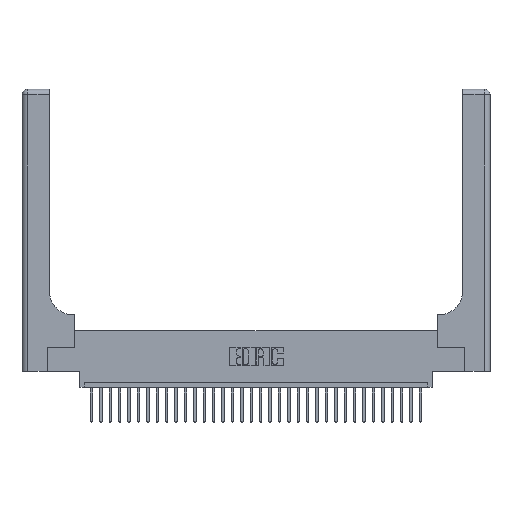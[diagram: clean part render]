
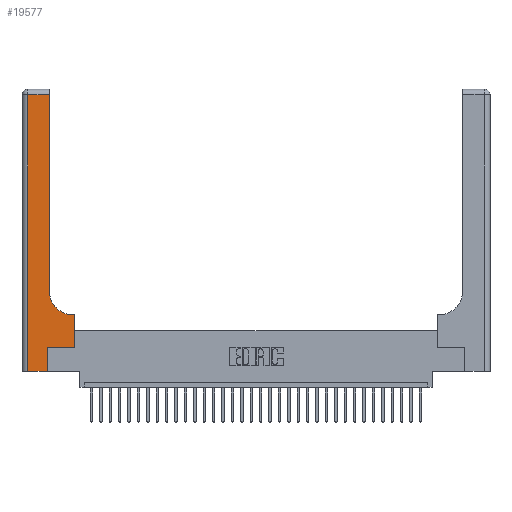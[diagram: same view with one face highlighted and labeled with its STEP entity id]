
A CAD part, top view. The second image highlights one B-rep face of the part: STEP entity #19577.
In plain terms, the highlighted planar face has unit normal (0, 0, 1).
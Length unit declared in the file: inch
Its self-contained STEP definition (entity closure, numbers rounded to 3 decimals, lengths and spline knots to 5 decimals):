
#452 = CARTESIAN_POINT ( 'NONE',  ( 0.5415, 0.6, 0.37 ) ) ;
#463 = VERTEX_POINT ( 'NONE', #10119 ) ;
#527 = CARTESIAN_POINT ( 'NONE',  ( 0.2915, 0.85, 0.37 ) ) ;
#620 = LINE ( 'NONE', #13643, #3871 ) ;
#786 = CARTESIAN_POINT ( 'NONE',  ( 0., 0., 0.37 ) ) ;
#1481 = LINE ( 'NONE', #9128, #20385 ) ;
#1831 = EDGE_CURVE ( 'NONE', #19878, #11481, #620, .T. ) ;
#1938 = CARTESIAN_POINT ( 'NONE',  ( 0.269, 0.25, 0.37 ) ) ;
#2171 = DIRECTION ( 'NONE',  ( 1., 0., 0. ) ) ;
#2666 = ORIENTED_EDGE ( 'NONE', *, *, #7732, .T. ) ;
#2807 = VECTOR ( 'NONE', #29113, 39.37008 ) ;
#3871 = VECTOR ( 'NONE', #11151, 39.37008 ) ;
#4984 = CIRCLE ( 'NONE', #26012, 0.25 ) ;
#5066 = LINE ( 'NONE', #786, #33152 ) ;
#5218 = DIRECTION ( 'NONE',  ( -1., 0., 0. ) ) ;
#6144 = VECTOR ( 'NONE', #14206, 39.37008 ) ;
#7732 = EDGE_CURVE ( 'NONE', #9405, #19878, #31428, .T. ) ;
#7807 = DIRECTION ( 'NONE',  ( 0., 0., -1. ) ) ;
#8270 = EDGE_CURVE ( 'NONE', #23010, #9405, #9745, .T. ) ;
#8709 = EDGE_CURVE ( 'NONE', #11481, #463, #5066, .T. ) ;
#9128 = CARTESIAN_POINT ( 'NONE',  ( 0.5585, 0.25, 0.37 ) ) ;
#9405 = VERTEX_POINT ( 'NONE', #33171 ) ;
#9745 = LINE ( 'NONE', #11195, #2807 ) ;
#10119 = CARTESIAN_POINT ( 'NONE',  ( 0.269, 0., 0.37 ) ) ;
#10226 = EDGE_CURVE ( 'NONE', #18715, #23010, #4984, .T. ) ;
#10331 = PLANE ( 'NONE',  #28315 ) ;
#10439 = ORIENTED_EDGE ( 'NONE', *, *, #27239, .T. ) ;
#11151 = DIRECTION ( 'NONE',  ( 0., -1., 0. ) ) ;
#11195 = CARTESIAN_POINT ( 'NONE',  ( 0.2915, 3., 0.37 ) ) ;
#11481 = VERTEX_POINT ( 'NONE', #20960 ) ;
#12913 = ORIENTED_EDGE ( 'NONE', *, *, #24461, .T. ) ;
#13223 = LINE ( 'NONE', #31880, #21623 ) ;
#13295 = ORIENTED_EDGE ( 'NONE', *, *, #23652, .T. ) ;
#13319 = CARTESIAN_POINT ( 'NONE',  ( 0.269, 0.25, 0.37 ) ) ;
#13643 = CARTESIAN_POINT ( 'NONE',  ( 0.06, 3., 0.37 ) ) ;
#14206 = DIRECTION ( 'NONE',  ( -1., 0., 0. ) ) ;
#14352 = EDGE_CURVE ( 'NONE', #16293, #25494, #1481, .T. ) ;
#15084 = CARTESIAN_POINT ( 'NONE',  ( 0.5585, 0.6, 0.37 ) ) ;
#15350 = ORIENTED_EDGE ( 'NONE', *, *, #10226, .T. ) ;
#15387 = EDGE_LOOP ( 'NONE', ( #16786, #2666, #30426, #17628, #10439, #12913, #19989, #13295, #15350 ) ) ;
#16293 = VERTEX_POINT ( 'NONE', #30199 ) ;
#16786 = ORIENTED_EDGE ( 'NONE', *, *, #8270, .T. ) ;
#16866 = CARTESIAN_POINT ( 'NONE',  ( 0., 2.94, 0.37 ) ) ;
#17628 = ORIENTED_EDGE ( 'NONE', *, *, #8709, .T. ) ;
#17678 = CARTESIAN_POINT ( 'NONE',  ( 0.06, 2.94, 0.37 ) ) ;
#18127 = FACE_OUTER_BOUND ( 'NONE', #15387, .T. ) ;
#18715 = VERTEX_POINT ( 'NONE', #452 ) ;
#19284 = CARTESIAN_POINT ( 'NONE',  ( 0.5415, 0.85, 0.37 ) ) ;
#19577 = ADVANCED_FACE ( 'NONE', ( #18127 ), #10331, .F. ) ;
#19878 = VERTEX_POINT ( 'NONE', #17678 ) ;
#19989 = ORIENTED_EDGE ( 'NONE', *, *, #14352, .T. ) ;
#20385 = VECTOR ( 'NONE', #22114, 39.37008 ) ;
#20569 = CARTESIAN_POINT ( 'NONE',  ( 0., 3., 0.37 ) ) ;
#20960 = CARTESIAN_POINT ( 'NONE',  ( 0.06, 0., 0.37 ) ) ;
#21623 = VECTOR ( 'NONE', #26392, 39.37008 ) ;
#21866 = DIRECTION ( 'NONE',  ( 0., 0., -1. ) ) ;
#22114 = DIRECTION ( 'NONE',  ( 0., 1., 0. ) ) ;
#22216 = LINE ( 'NONE', #13319, #23031 ) ;
#23010 = VERTEX_POINT ( 'NONE', #527 ) ;
#23031 = VECTOR ( 'NONE', #26514, 39.37008 ) ;
#23652 = EDGE_CURVE ( 'NONE', #25494, #18715, #28240, .T. ) ;
#24461 = EDGE_CURVE ( 'NONE', #31440, #16293, #22216, .T. ) ;
#25494 = VERTEX_POINT ( 'NONE', #15084 ) ;
#26012 = AXIS2_PLACEMENT_3D ( 'NONE', #19284, #21866, #2171 ) ;
#26392 = DIRECTION ( 'NONE',  ( 0., 1., 0. ) ) ;
#26514 = DIRECTION ( 'NONE',  ( 1., 0., 0. ) ) ;
#26657 = DIRECTION ( 'NONE',  ( -1., 0., 0. ) ) ;
#26867 = DIRECTION ( 'NONE',  ( 1., 0., 0. ) ) ;
#27239 = EDGE_CURVE ( 'NONE', #463, #31440, #13223, .T. ) ;
#28240 = LINE ( 'NONE', #32151, #30680 ) ;
#28315 = AXIS2_PLACEMENT_3D ( 'NONE', #20569, #7807, #5218 ) ;
#29113 = DIRECTION ( 'NONE',  ( 0., 1., 0. ) ) ;
#30199 = CARTESIAN_POINT ( 'NONE',  ( 0.5585, 0.25, 0.37 ) ) ;
#30426 = ORIENTED_EDGE ( 'NONE', *, *, #1831, .T. ) ;
#30680 = VECTOR ( 'NONE', #26657, 39.37008 ) ;
#31428 = LINE ( 'NONE', #16866, #6144 ) ;
#31440 = VERTEX_POINT ( 'NONE', #1938 ) ;
#31880 = CARTESIAN_POINT ( 'NONE',  ( 0.269, 0., 0.37 ) ) ;
#32151 = CARTESIAN_POINT ( 'NONE',  ( 0.2915, 0.6, 0.37 ) ) ;
#33152 = VECTOR ( 'NONE', #26867, 39.37008 ) ;
#33171 = CARTESIAN_POINT ( 'NONE',  ( 0.2915, 2.94, 0.37 ) ) ;
